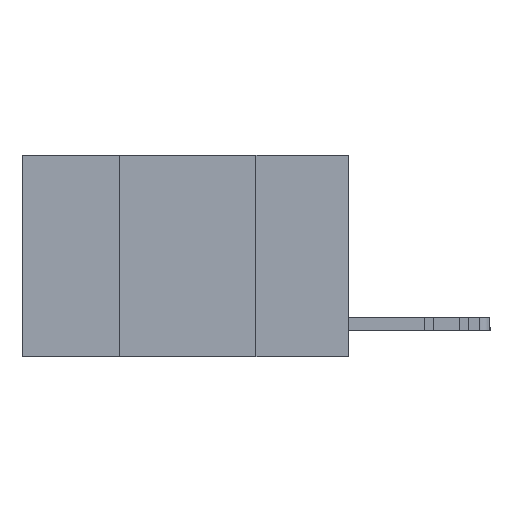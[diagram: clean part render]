
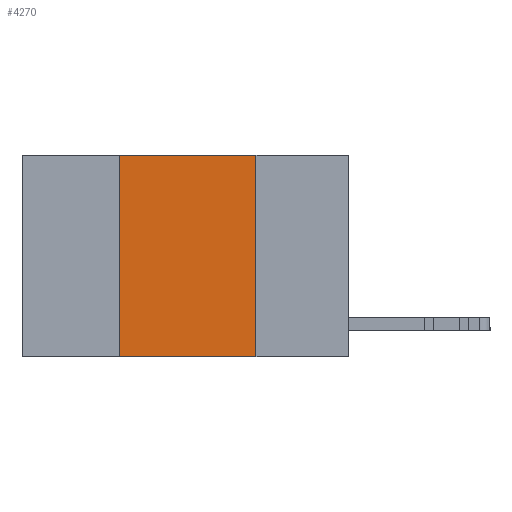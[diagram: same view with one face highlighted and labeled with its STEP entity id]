
A CAD part, left-side view. The second image highlights one B-rep face of the part: STEP entity #4270.
In plain terms, the highlighted planar face has unit normal (-1, 0, 0).
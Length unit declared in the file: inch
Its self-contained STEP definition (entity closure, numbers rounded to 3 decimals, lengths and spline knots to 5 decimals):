
#76 = CARTESIAN_POINT ( 'NONE',  ( 0., 0.42, -0.37 ) ) ;
#1074 = CARTESIAN_POINT ( 'NONE',  ( 0., 0.42, 0. ) ) ;
#2076 = DIRECTION ( 'NONE',  ( 0., -1., 0. ) ) ;
#2269 = VECTOR ( 'NONE', #11264, 39.37008 ) ;
#3514 = CARTESIAN_POINT ( 'NONE',  ( 0., 0.17, 0. ) ) ;
#4270 = ADVANCED_FACE ( 'NONE', ( #19332 ), #5066, .F. ) ;
#5066 = PLANE ( 'NONE',  #5818 ) ;
#5528 = CARTESIAN_POINT ( 'NONE',  ( 0., 0.6, -0.37 ) ) ;
#5678 = LINE ( 'NONE', #14302, #16897 ) ;
#5818 = AXIS2_PLACEMENT_3D ( 'NONE', #9076, #8939, #15226 ) ;
#5880 = VERTEX_POINT ( 'NONE', #76 ) ;
#6379 = VECTOR ( 'NONE', #7719, 39.37008 ) ;
#6831 = EDGE_CURVE ( 'NONE', #5880, #16234, #25778, .T. ) ;
#7719 = DIRECTION ( 'NONE',  ( 0., -1., 0. ) ) ;
#8490 = CARTESIAN_POINT ( 'NONE',  ( 0., 0.17, -0.37 ) ) ;
#8853 = EDGE_CURVE ( 'NONE', #22875, #14890, #13602, .T. ) ;
#8939 = DIRECTION ( 'NONE',  ( 1., 0., 0. ) ) ;
#8959 = EDGE_LOOP ( 'NONE', ( #9881, #19651, #21379, #19304 ) ) ;
#9076 = CARTESIAN_POINT ( 'NONE',  ( 0., 0.6, 0. ) ) ;
#9881 = ORIENTED_EDGE ( 'NONE', *, *, #8853, .F. ) ;
#11264 = DIRECTION ( 'NONE',  ( 0., 0., 1. ) ) ;
#12528 = EDGE_CURVE ( 'NONE', #16234, #22875, #5678, .T. ) ;
#13062 = CARTESIAN_POINT ( 'NONE',  ( 0., 0.42, 0. ) ) ;
#13602 = LINE ( 'NONE', #21943, #20316 ) ;
#14302 = CARTESIAN_POINT ( 'NONE',  ( 0., 0.6, 0. ) ) ;
#14890 = VERTEX_POINT ( 'NONE', #8490 ) ;
#15226 = DIRECTION ( 'NONE',  ( 0., 0., -1. ) ) ;
#16234 = VERTEX_POINT ( 'NONE', #13062 ) ;
#16897 = VECTOR ( 'NONE', #2076, 39.37008 ) ;
#19304 = ORIENTED_EDGE ( 'NONE', *, *, #25981, .T. ) ;
#19332 = FACE_OUTER_BOUND ( 'NONE', #8959, .T. ) ;
#19651 = ORIENTED_EDGE ( 'NONE', *, *, #12528, .F. ) ;
#20316 = VECTOR ( 'NONE', #21819, 39.37008 ) ;
#21379 = ORIENTED_EDGE ( 'NONE', *, *, #6831, .F. ) ;
#21819 = DIRECTION ( 'NONE',  ( 0., 0., -1. ) ) ;
#21943 = CARTESIAN_POINT ( 'NONE',  ( 0., 0.17, 0. ) ) ;
#22875 = VERTEX_POINT ( 'NONE', #3514 ) ;
#25778 = LINE ( 'NONE', #1074, #2269 ) ;
#25981 = EDGE_CURVE ( 'NONE', #5880, #14890, #26754, .T. ) ;
#26754 = LINE ( 'NONE', #5528, #6379 ) ;
